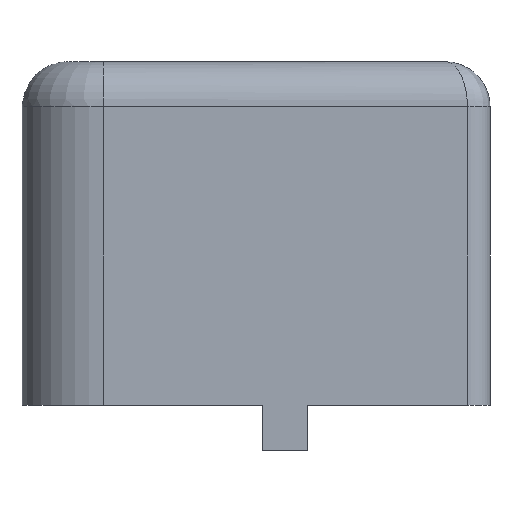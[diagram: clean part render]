
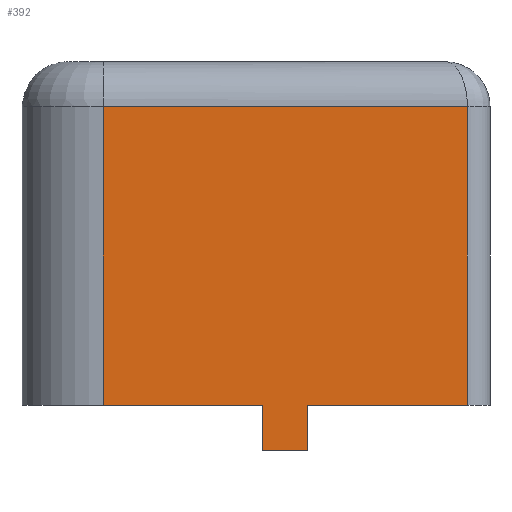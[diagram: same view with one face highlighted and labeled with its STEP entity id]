
A CAD part, left-side view. The second image highlights one B-rep face of the part: STEP entity #392.
In plain terms, the highlighted planar face has unit normal (-1, 0, 0).
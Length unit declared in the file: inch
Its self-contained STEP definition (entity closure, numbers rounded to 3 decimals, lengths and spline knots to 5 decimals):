
#21 = EDGE_CURVE ( 'NONE', #1559, #1518, #824, .T. ) ;
#64 = CARTESIAN_POINT ( 'NONE',  ( -0.76802, -0.06467, -0.3937 ) ) ;
#76 = VERTEX_POINT ( 'NONE', #1341 ) ;
#154 = DIRECTION ( 'NONE',  ( 1., 0., 0. ) ) ;
#162 = CARTESIAN_POINT ( 'NONE',  ( -0.76802, 1.32953, 0.03937 ) ) ;
#167 = DIRECTION ( 'NONE',  ( 0., 1., 0. ) ) ;
#203 = AXIS2_PLACEMENT_3D ( 'NONE', #1282, #154, #1044 ) ;
#251 = VERTEX_POINT ( 'NONE', #401 ) ;
#257 = VECTOR ( 'NONE', #308, 39.37008 ) ;
#300 = LINE ( 'NONE', #937, #257 ) ;
#303 = CARTESIAN_POINT ( 'NONE',  ( -0.76802, 1.32953, 2.6063 ) ) ;
#308 = DIRECTION ( 'NONE',  ( 0., -1., 0. ) ) ;
#314 = CARTESIAN_POINT ( 'NONE',  ( -0.76802, -0.45838, -0.3937 ) ) ;
#319 = DIRECTION ( 'NONE',  ( 0., -1., 0. ) ) ;
#339 = LINE ( 'NONE', #673, #1295 ) ;
#375 = LINE ( 'NONE', #162, #1006 ) ;
#392 = ADVANCED_FACE ( 'NONE', ( #1028 ), #1534, .F. ) ;
#401 = CARTESIAN_POINT ( 'NONE',  ( -0.76802, 1.32953, 2.6063 ) ) ;
#423 = CARTESIAN_POINT ( 'NONE',  ( -0.76802, -0.45838, 0. ) ) ;
#439 = CARTESIAN_POINT ( 'NONE',  ( -0.76802, -0.45838, -0.3937 ) ) ;
#448 = VERTEX_POINT ( 'NONE', #1415 ) ;
#453 = ORIENTED_EDGE ( 'NONE', *, *, #828, .T. ) ;
#485 = VECTOR ( 'NONE', #584, 39.37008 ) ;
#551 = CARTESIAN_POINT ( 'NONE',  ( -0.76802, -0.06467, 0. ) ) ;
#554 = CARTESIAN_POINT ( 'NONE',  ( -0.76802, 1.32953, 0. ) ) ;
#584 = DIRECTION ( 'NONE',  ( 0., 0., 1. ) ) ;
#595 = VECTOR ( 'NONE', #319, 39.37008 ) ;
#613 = VERTEX_POINT ( 'NONE', #439 ) ;
#634 = VECTOR ( 'NONE', #167, 39.37008 ) ;
#673 = CARTESIAN_POINT ( 'NONE',  ( -0.76802, -1.85258, 0.03937 ) ) ;
#686 = CARTESIAN_POINT ( 'NONE',  ( -0.76802, 1.32953, 0. ) ) ;
#713 = ORIENTED_EDGE ( 'NONE', *, *, #816, .T. ) ;
#724 = ORIENTED_EDGE ( 'NONE', *, *, #840, .T. ) ;
#729 = EDGE_CURVE ( 'NONE', #251, #1399, #375, .T. ) ;
#773 = EDGE_CURVE ( 'NONE', #76, #448, #339, .T. ) ;
#786 = EDGE_CURVE ( 'NONE', #76, #251, #1624, .T. ) ;
#798 = EDGE_CURVE ( 'NONE', #1399, #1518, #1591, .T. ) ;
#816 = EDGE_CURVE ( 'NONE', #1559, #613, #300, .T. ) ;
#824 = LINE ( 'NONE', #64, #485 ) ;
#828 = EDGE_CURVE ( 'NONE', #613, #1500, #890, .T. ) ;
#840 = EDGE_CURVE ( 'NONE', #1500, #448, #1511, .T. ) ;
#852 = EDGE_LOOP ( 'NONE', ( #898, #1540, #1141, #1245, #965, #713, #453, #724 ) ) ;
#890 = LINE ( 'NONE', #314, #932 ) ;
#898 = ORIENTED_EDGE ( 'NONE', *, *, #773, .F. ) ;
#927 = DIRECTION ( 'NONE',  ( 0., 0., -1. ) ) ;
#932 = VECTOR ( 'NONE', #1186, 39.37008 ) ;
#935 = CARTESIAN_POINT ( 'NONE',  ( -0.76802, -0.06467, -0.3937 ) ) ;
#937 = CARTESIAN_POINT ( 'NONE',  ( -0.76802, -0.06467, -0.3937 ) ) ;
#965 = ORIENTED_EDGE ( 'NONE', *, *, #21, .F. ) ;
#1006 = VECTOR ( 'NONE', #927, 39.37008 ) ;
#1028 = FACE_OUTER_BOUND ( 'NONE', #852, .T. ) ;
#1044 = DIRECTION ( 'NONE',  ( 0., 0., -1. ) ) ;
#1061 = DIRECTION ( 'NONE',  ( 0., -1., 0. ) ) ;
#1074 = CARTESIAN_POINT ( 'NONE',  ( -0.76802, -0.45838, 0. ) ) ;
#1141 = ORIENTED_EDGE ( 'NONE', *, *, #729, .T. ) ;
#1186 = DIRECTION ( 'NONE',  ( 0., 0., 1. ) ) ;
#1245 = ORIENTED_EDGE ( 'NONE', *, *, #798, .T. ) ;
#1252 = VECTOR ( 'NONE', #1061, 39.37008 ) ;
#1282 = CARTESIAN_POINT ( 'NONE',  ( -0.76802, -0.45838, 0.03937 ) ) ;
#1295 = VECTOR ( 'NONE', #1546, 39.37008 ) ;
#1341 = CARTESIAN_POINT ( 'NONE',  ( -0.76802, -1.85258, 2.6063 ) ) ;
#1399 = VERTEX_POINT ( 'NONE', #686 ) ;
#1415 = CARTESIAN_POINT ( 'NONE',  ( -0.76802, -1.85258, 0. ) ) ;
#1500 = VERTEX_POINT ( 'NONE', #423 ) ;
#1511 = LINE ( 'NONE', #1074, #595 ) ;
#1518 = VERTEX_POINT ( 'NONE', #551 ) ;
#1534 = PLANE ( 'NONE',  #203 ) ;
#1540 = ORIENTED_EDGE ( 'NONE', *, *, #786, .T. ) ;
#1546 = DIRECTION ( 'NONE',  ( 0., 0., -1. ) ) ;
#1559 = VERTEX_POINT ( 'NONE', #935 ) ;
#1591 = LINE ( 'NONE', #554, #1252 ) ;
#1624 = LINE ( 'NONE', #303, #634 ) ;
